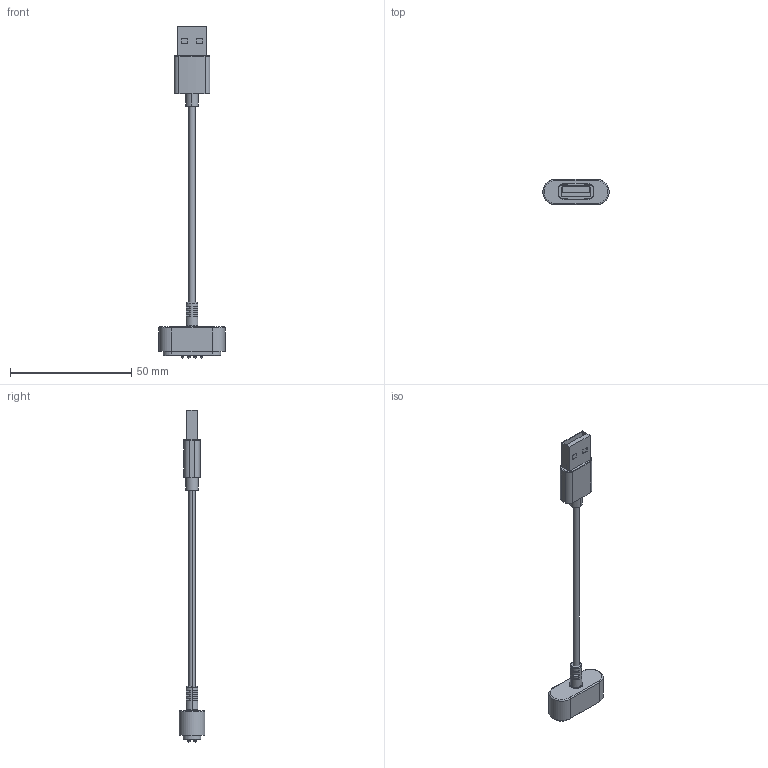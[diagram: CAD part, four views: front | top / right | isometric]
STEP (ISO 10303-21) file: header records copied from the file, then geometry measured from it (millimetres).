
FILE_DESCRIPTION (( 'STEP AP214' ), '1' );
FILE_NAME ('687B0812A512100.STEP', '2023-04-13T16:20:32', ( '' ), ( '' ), 'SwSTEP 2.0', 'SolidWorks 2020', '' );
FILE_SCHEMA (( 'AUTOMOTIVE_DESIGN' ));
Length unit declared in the file: millimetre
Products named in the file (1): 687B0812A512100
Bounding box: 27.3 x 10.6 x 136.9 mm (x, y, z)
Volume: 4444.9 mm3; surface area: 5288 mm2
Topology: 11 solids, 12 shells, 523 faces, 1263 edges, 814 vertices
Faces by surface type: plane 258, cylinder 137, torus 54, cone 40, bspline 18, sphere 16
Entity records: 18096 total; most frequent: CARTESIAN_POINT 6296, ORIENTED_EDGE 2494, DIRECTION 1968, EDGE_CURVE 1247, VERTEX_POINT 814, AXIS2_PLACEMENT_3D 696, EDGE_LOOP 595, VECTOR 576
